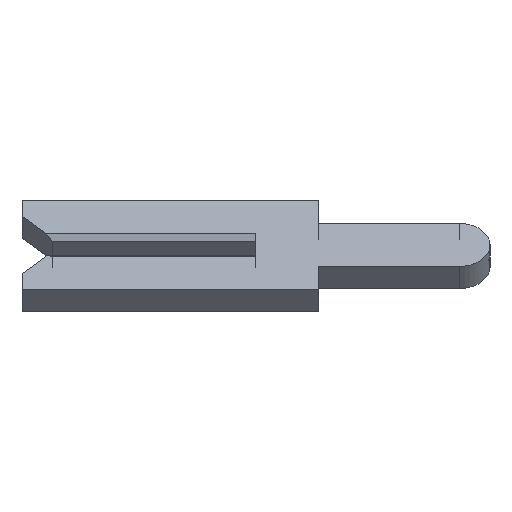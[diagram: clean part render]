
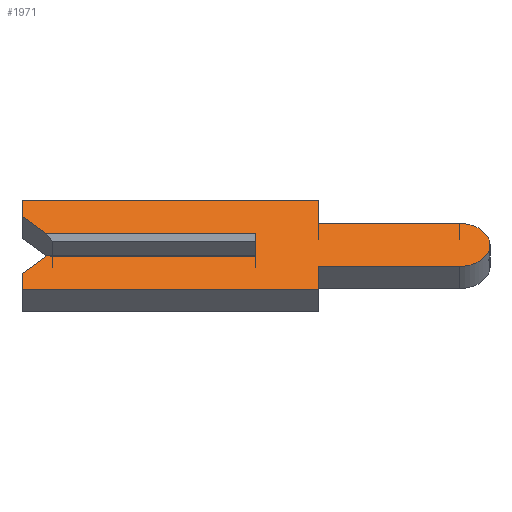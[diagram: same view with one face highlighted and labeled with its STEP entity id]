
A CAD part, left-side view. The second image highlights one B-rep face of the part: STEP entity #1971.
In plain terms, the highlighted face is planar.
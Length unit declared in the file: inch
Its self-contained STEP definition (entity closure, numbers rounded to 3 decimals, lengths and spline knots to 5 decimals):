
#9 = VECTOR ( 'NONE', #562, 39.37008 ) ;
#51 = CARTESIAN_POINT ( 'NONE',  ( -0.01, -0.1305, 0.0195 ) ) ;
#79 = DIRECTION ( 'NONE',  ( 0., 0., 1. ) ) ;
#93 = VECTOR ( 'NONE', #2064, 39.37008 ) ;
#97 = ORIENTED_EDGE ( 'NONE', *, *, #981, .F. ) ;
#127 = LINE ( 'NONE', #1790, #1074 ) ;
#176 = CARTESIAN_POINT ( 'NONE',  ( -0.01, -0.1305, -0.0195 ) ) ;
#181 = VERTEX_POINT ( 'NONE', #611 ) ;
#223 = CARTESIAN_POINT ( 'NONE',  ( -0.01, 0.15, -0.026 ) ) ;
#272 = DIRECTION ( 'NONE',  ( 0., -0.707, 0.707 ) ) ;
#282 = ORIENTED_EDGE ( 'NONE', *, *, #574, .F. ) ;
#300 = VECTOR ( 'NONE', #1236, 39.37008 ) ;
#323 = ORIENTED_EDGE ( 'NONE', *, *, #646, .F. ) ;
#330 = LINE ( 'NONE', #223, #441 ) ;
#366 = CARTESIAN_POINT ( 'NONE',  ( -0.01, 0.134, -0.01 ) ) ;
#379 = DIRECTION ( 'NONE',  ( 1., 0., 0. ) ) ;
#384 = CARTESIAN_POINT ( 'NONE',  ( -0.01, -0.1305, 0. ) ) ;
#405 = ORIENTED_EDGE ( 'NONE', *, *, #605, .F. ) ;
#414 = CIRCLE ( 'NONE', #1142, 0.0195 ) ;
#431 = ORIENTED_EDGE ( 'NONE', *, *, #786, .T. ) ;
#433 = CARTESIAN_POINT ( 'NONE',  ( -0.01, -0.04, 0.0195 ) ) ;
#441 = VECTOR ( 'NONE', #1164, 39.37008 ) ;
#449 = ORIENTED_EDGE ( 'NONE', *, *, #1625, .F. ) ;
#468 = CARTESIAN_POINT ( 'NONE',  ( -0.01, -0.04, -0.04 ) ) ;
#472 = VERTEX_POINT ( 'NONE', #1614 ) ;
#479 = VECTOR ( 'NONE', #2395, 39.37008 ) ;
#519 = CARTESIAN_POINT ( 'NONE',  ( -0.01, 0.1305, 0.0065 ) ) ;
#562 = DIRECTION ( 'NONE',  ( 0., 1., 0. ) ) ;
#574 = EDGE_CURVE ( 'NONE', #2376, #1229, #718, .T. ) ;
#578 = VERTEX_POINT ( 'NONE', #831 ) ;
#585 = CARTESIAN_POINT ( 'NONE',  ( -0.01, 0.15, -0.04 ) ) ;
#595 = VECTOR ( 'NONE', #669, 39.37008 ) ;
#605 = EDGE_CURVE ( 'NONE', #1586, #181, #2088, .T. ) ;
#608 = ORIENTED_EDGE ( 'NONE', *, *, #696, .F. ) ;
#611 = CARTESIAN_POINT ( 'NONE',  ( -0.01, -0.04, 0.04 ) ) ;
#624 = LINE ( 'NONE', #468, #300 ) ;
#637 = DIRECTION ( 'NONE',  ( 0., -1., 0. ) ) ;
#646 = EDGE_CURVE ( 'NONE', #1343, #472, #684, .T. ) ;
#669 = DIRECTION ( 'NONE',  ( 0., 0., 1. ) ) ;
#684 = LINE ( 'NONE', #1634, #1713 ) ;
#696 = EDGE_CURVE ( 'NONE', #1832, #1080, #624, .T. ) ;
#718 = LINE ( 'NONE', #1194, #1445 ) ;
#732 = CARTESIAN_POINT ( 'NONE',  ( -0.01, 0., -0.01 ) ) ;
#757 = CARTESIAN_POINT ( 'NONE',  ( -0.01, -0.1305, 0. ) ) ;
#786 = EDGE_CURVE ( 'NONE', #2016, #472, #127, .T. ) ;
#831 = CARTESIAN_POINT ( 'NONE',  ( -0.01, 0.15, 0.026 ) ) ;
#943 = EDGE_CURVE ( 'NONE', #578, #1586, #1632, .T. ) ;
#981 = EDGE_CURVE ( 'NONE', #1229, #1343, #1596, .T. ) ;
#1007 = LINE ( 'NONE', #1910, #1991 ) ;
#1025 = EDGE_CURVE ( 'NONE', #2016, #578, #2083, .T. ) ;
#1039 = VECTOR ( 'NONE', #1851, 39.37008 ) ;
#1060 = CARTESIAN_POINT ( 'NONE',  ( -0.01, -0.1305, -0.01 ) ) ;
#1064 = ORIENTED_EDGE ( 'NONE', *, *, #1544, .F. ) ;
#1066 = AXIS2_PLACEMENT_3D ( 'NONE', #757, #379, #1925 ) ;
#1074 = VECTOR ( 'NONE', #637, 39.37008 ) ;
#1080 = VERTEX_POINT ( 'NONE', #2422 ) ;
#1104 = LINE ( 'NONE', #433, #1218 ) ;
#1123 = DIRECTION ( 'NONE',  ( 0., 0., -1. ) ) ;
#1142 = AXIS2_PLACEMENT_3D ( 'NONE', #384, #1942, #1123 ) ;
#1151 = CARTESIAN_POINT ( 'NONE',  ( -0.01, -0.04, -0.0195 ) ) ;
#1154 = LINE ( 'NONE', #1698, #1953 ) ;
#1164 = DIRECTION ( 'NONE',  ( 0., 0., 1. ) ) ;
#1188 = CARTESIAN_POINT ( 'NONE',  ( -0.01, 0.134, 0.01 ) ) ;
#1194 = CARTESIAN_POINT ( 'NONE',  ( -0.01, 0.1305, -0.0065 ) ) ;
#1218 = VECTOR ( 'NONE', #2153, 39.37008 ) ;
#1229 = VERTEX_POINT ( 'NONE', #366 ) ;
#1236 = DIRECTION ( 'NONE',  ( 0., 0., -1. ) ) ;
#1277 = ORIENTED_EDGE ( 'NONE', *, *, #943, .F. ) ;
#1298 = VERTEX_POINT ( 'NONE', #2091 ) ;
#1343 = VERTEX_POINT ( 'NONE', #732 ) ;
#1401 = ORIENTED_EDGE ( 'NONE', *, *, #2178, .F. ) ;
#1406 = CARTESIAN_POINT ( 'NONE',  ( -0.01, 0.15, 0.04 ) ) ;
#1411 = LINE ( 'NONE', #1509, #9 ) ;
#1445 = VECTOR ( 'NONE', #272, 39.37008 ) ;
#1488 = DIRECTION ( 'NONE',  ( 0., 0., -1. ) ) ;
#1509 = CARTESIAN_POINT ( 'NONE',  ( -0.01, -0.04, -0.0195 ) ) ;
#1524 = EDGE_CURVE ( 'NONE', #1611, #1832, #1411, .T. ) ;
#1531 = PLANE ( 'NONE',  #1066 ) ;
#1544 = EDGE_CURVE ( 'NONE', #181, #1298, #1154, .T. ) ;
#1565 = ORIENTED_EDGE ( 'NONE', *, *, #1524, .F. ) ;
#1586 = VERTEX_POINT ( 'NONE', #1889 ) ;
#1596 = LINE ( 'NONE', #1060, #1039 ) ;
#1611 = VERTEX_POINT ( 'NONE', #176 ) ;
#1614 = CARTESIAN_POINT ( 'NONE',  ( -0.01, 0., 0.01 ) ) ;
#1625 = EDGE_CURVE ( 'NONE', #1080, #1762, #1007, .T. ) ;
#1632 = LINE ( 'NONE', #2440, #595 ) ;
#1634 = CARTESIAN_POINT ( 'NONE',  ( -0.01, 0., 0.0065 ) ) ;
#1647 = EDGE_CURVE ( 'NONE', #2052, #1611, #414, .T. ) ;
#1698 = CARTESIAN_POINT ( 'NONE',  ( -0.01, -0.04, 0.04 ) ) ;
#1713 = VECTOR ( 'NONE', #79, 39.37008 ) ;
#1733 = DIRECTION ( 'NONE',  ( 0., 1., 0. ) ) ;
#1749 = ORIENTED_EDGE ( 'NONE', *, *, #1025, .F. ) ;
#1762 = VERTEX_POINT ( 'NONE', #585 ) ;
#1790 = CARTESIAN_POINT ( 'NONE',  ( -0.01, 0.15, 0.01 ) ) ;
#1832 = VERTEX_POINT ( 'NONE', #1151 ) ;
#1851 = DIRECTION ( 'NONE',  ( 0., -1., 0. ) ) ;
#1889 = CARTESIAN_POINT ( 'NONE',  ( -0.01, 0.15, 0.04 ) ) ;
#1903 = ORIENTED_EDGE ( 'NONE', *, *, #1647, .F. ) ;
#1910 = CARTESIAN_POINT ( 'NONE',  ( -0.01, 0.15, -0.04 ) ) ;
#1925 = DIRECTION ( 'NONE',  ( 0., 0., -1. ) ) ;
#1942 = DIRECTION ( 'NONE',  ( 1., 0., 0. ) ) ;
#1953 = VECTOR ( 'NONE', #1488, 39.37008 ) ;
#1971 = ADVANCED_FACE ( 'NONE', ( #2325 ), #1531, .F. ) ;
#1991 = VECTOR ( 'NONE', #1733, 39.37008 ) ;
#2016 = VERTEX_POINT ( 'NONE', #1188 ) ;
#2052 = VERTEX_POINT ( 'NONE', #51 ) ;
#2064 = DIRECTION ( 'NONE',  ( 0., 0.707, 0.707 ) ) ;
#2083 = LINE ( 'NONE', #519, #93 ) ;
#2088 = LINE ( 'NONE', #1406, #479 ) ;
#2091 = CARTESIAN_POINT ( 'NONE',  ( -0.01, -0.04, 0.0195 ) ) ;
#2153 = DIRECTION ( 'NONE',  ( 0., -1., 0. ) ) ;
#2178 = EDGE_CURVE ( 'NONE', #1298, #2052, #1104, .T. ) ;
#2255 = EDGE_LOOP ( 'NONE', ( #431, #323, #97, #282, #2341, #449, #608, #1565, #1903, #1401, #1064, #405, #1277, #1749 ) ) ;
#2325 = FACE_OUTER_BOUND ( 'NONE', #2255, .T. ) ;
#2339 = EDGE_CURVE ( 'NONE', #1762, #2376, #330, .T. ) ;
#2341 = ORIENTED_EDGE ( 'NONE', *, *, #2339, .F. ) ;
#2354 = CARTESIAN_POINT ( 'NONE',  ( -0.01, 0.15, -0.026 ) ) ;
#2376 = VERTEX_POINT ( 'NONE', #2354 ) ;
#2395 = DIRECTION ( 'NONE',  ( 0., -1., 0. ) ) ;
#2422 = CARTESIAN_POINT ( 'NONE',  ( -0.01, -0.04, -0.04 ) ) ;
#2440 = CARTESIAN_POINT ( 'NONE',  ( -0.01, 0.15, 0.026 ) ) ;
